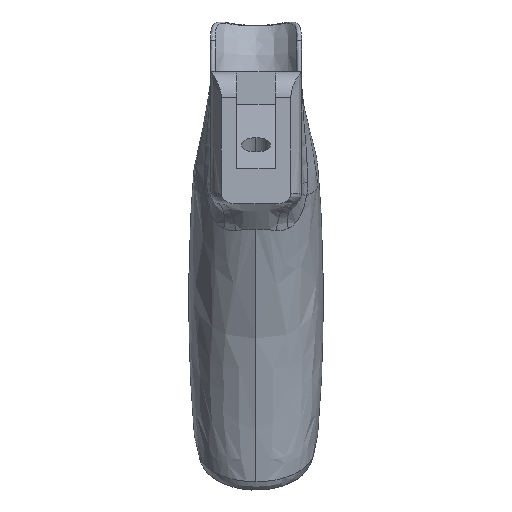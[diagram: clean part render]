
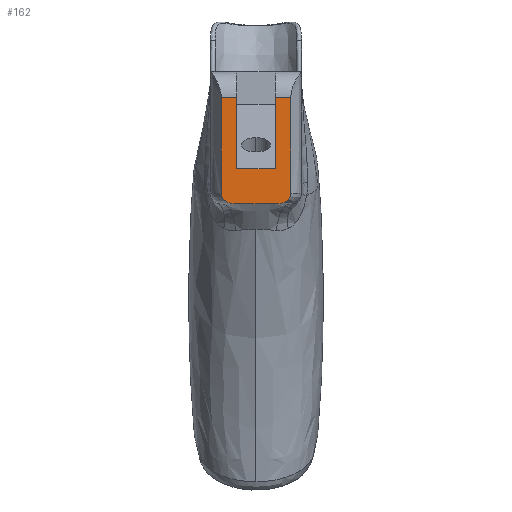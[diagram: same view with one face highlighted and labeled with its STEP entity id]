
A CAD part, top view. The second image highlights one B-rep face of the part: STEP entity #162.
In plain terms, the highlighted planar face has unit normal (0, 0, 1).
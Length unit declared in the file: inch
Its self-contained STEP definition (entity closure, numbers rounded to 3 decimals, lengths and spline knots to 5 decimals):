
#19 = VECTOR ( 'NONE', #7024, 39.37008 ) ;
#74 = CARTESIAN_POINT ( 'NONE',  ( -0.24455, -1.27484, 0. ) ) ;
#162 = ADVANCED_FACE ( 'NONE', ( #7116 ), #1725, .T. ) ;
#166 = VECTOR ( 'NONE', #4047, 39.37008 ) ;
#286 = CARTESIAN_POINT ( 'NONE',  ( 0.3375, -1.1789, 0. ) ) ;
#316 = VECTOR ( 'NONE', #1721, 39.37008 ) ;
#456 = DIRECTION ( 'NONE',  ( 0., 1., 0. ) ) ;
#489 = CARTESIAN_POINT ( 'NONE',  ( -0.188, -0.94, 0. ) ) ;
#516 = CARTESIAN_POINT ( 'NONE',  ( -0.188, -0.25, 0. ) ) ;
#560 = CARTESIAN_POINT ( 'NONE',  ( -0.26647, -1.26868, 0. ) ) ;
#705 = ORIENTED_EDGE ( 'NONE', *, *, #6036, .T. ) ;
#712 = CARTESIAN_POINT ( 'NONE',  ( -0.2069, -1.2789, 0. ) ) ;
#732 = CARTESIAN_POINT ( 'NONE',  ( 0.3208, -1.22844, 0. ) ) ;
#767 = ORIENTED_EDGE ( 'NONE', *, *, #5271, .F. ) ;
#1080 = DIRECTION ( 'NONE',  ( 1., 0., 0. ) ) ;
#1212 = LINE ( 'NONE', #3583, #316 ) ;
#1233 = CARTESIAN_POINT ( 'NONE',  ( -0.32073, -1.22843, 0. ) ) ;
#1303 = CARTESIAN_POINT ( 'NONE',  ( -0.30517, -1.2451, 0. ) ) ;
#1326 = CARTESIAN_POINT ( 'NONE',  ( 0.30534, -1.24507, 0. ) ) ;
#1360 = B_SPLINE_CURVE_WITH_KNOTS ( 'NONE', 3,
 ( #3565, #4887, #5471, #6614, #1813, #1233, #4848, #1303, #6647, #5400, #560, #74, #1739, #2376, #5361, #6543 ),
 .UNSPECIFIED., .F., .F.,
 ( 4, 2, 2, 2, 2, 2, 2, 4 ),
 ( 0., 0.00058, 0.00115, 0.00173, 0.0023, 0.00345, 0.00403, 0.0046 ),
 .UNSPECIFIED. ) ;
#1496 = CARTESIAN_POINT ( 'NONE',  ( -0.3375, -0.25, 0. ) ) ;
#1583 = ORIENTED_EDGE ( 'NONE', *, *, #2673, .F. ) ;
#1663 = VECTOR ( 'NONE', #2103, 39.37008 ) ;
#1671 = LINE ( 'NONE', #3535, #6327 ) ;
#1673 = VERTEX_POINT ( 'NONE', #2850 ) ;
#1721 = DIRECTION ( 'NONE',  ( 0., 1., 0. ) ) ;
#1725 = PLANE ( 'NONE',  #7564 ) ;
#1739 = CARTESIAN_POINT ( 'NONE',  ( -0.23707, -1.27637, 0. ) ) ;
#1784 = DIRECTION ( 'NONE',  ( 0., -1., 0. ) ) ;
#1805 = VECTOR ( 'NONE', #456, 39.37008 ) ;
#1813 = CARTESIAN_POINT ( 'NONE',  ( -0.32875, -1.21558, 0. ) ) ;
#1836 = DIRECTION ( 'NONE',  ( 0., -1., 0. ) ) ;
#1981 = CARTESIAN_POINT ( 'NONE',  ( 0.22262, -1.2789, 0. ) ) ;
#2103 = DIRECTION ( 'NONE',  ( 0., -1., 0. ) ) ;
#2192 = CARTESIAN_POINT ( 'NONE',  ( 0.20741, -1.2789, 0. ) ) ;
#2229 = ORIENTED_EDGE ( 'NONE', *, *, #2868, .F. ) ;
#2259 = LINE ( 'NONE', #7051, #6829 ) ;
#2285 = CARTESIAN_POINT ( 'NONE',  ( 0.3375, -0.25, 0. ) ) ;
#2314 = B_SPLINE_CURVE_WITH_KNOTS ( 'NONE', 3,
 ( #7379, #1981, #3261, #5649, #4285, #4906, #6710, #7295, #1326, #3735, #732, #3146, #5529, #2773, #5128, #286 ),
 .UNSPECIFIED., .F., .F.,
 ( 4, 2, 2, 2, 2, 2, 2, 4 ),
 ( 0., 0.00115, 0.00172, 0.00229, 0.00286, 0.00344, 0.00401, 0.00458 ),
 .UNSPECIFIED. ) ;
#2348 = CARTESIAN_POINT ( 'NONE',  ( 0.187, 0., 0. ) ) ;
#2376 = CARTESIAN_POINT ( 'NONE',  ( -0.22208, -1.27839, 0. ) ) ;
#2386 = DIRECTION ( 'NONE',  ( 1., 0., 0. ) ) ;
#2620 = ORIENTED_EDGE ( 'NONE', *, *, #2959, .T. ) ;
#2673 = EDGE_CURVE ( 'NONE', #3401, #3157, #5133, .T. ) ;
#2768 = VERTEX_POINT ( 'NONE', #2192 ) ;
#2773 = CARTESIAN_POINT ( 'NONE',  ( 0.33636, -1.19408, 0. ) ) ;
#2813 = VECTOR ( 'NONE', #1784, 39.37008 ) ;
#2850 = CARTESIAN_POINT ( 'NONE',  ( 0.187, -0.25, 0. ) ) ;
#2868 = EDGE_CURVE ( 'NONE', #1673, #3878, #5769, .T. ) ;
#2959 = EDGE_CURVE ( 'NONE', #4419, #3878, #5731, .T. ) ;
#3146 = CARTESIAN_POINT ( 'NONE',  ( 0.3288, -1.21555, 0. ) ) ;
#3157 = VERTEX_POINT ( 'NONE', #3578 ) ;
#3261 = CARTESIAN_POINT ( 'NONE',  ( 0.23752, -1.27691, 0. ) ) ;
#3335 = VERTEX_POINT ( 'NONE', #1496 ) ;
#3401 = VERTEX_POINT ( 'NONE', #516 ) ;
#3461 = CARTESIAN_POINT ( 'NONE',  ( -0.188, 0., 0. ) ) ;
#3535 = CARTESIAN_POINT ( 'NONE',  ( -0.4425, -0.25, 0. ) ) ;
#3565 = CARTESIAN_POINT ( 'NONE',  ( -0.3375, -1.1789, 0. ) ) ;
#3578 = CARTESIAN_POINT ( 'NONE',  ( -0.188, -0.94, 0. ) ) ;
#3583 = CARTESIAN_POINT ( 'NONE',  ( -0.3375, -1.2789, 0. ) ) ;
#3590 = CARTESIAN_POINT ( 'NONE',  ( -0.4425, -0.25, 0. ) ) ;
#3735 = CARTESIAN_POINT ( 'NONE',  ( 0.31598, -1.2344, 0. ) ) ;
#3784 = VERTEX_POINT ( 'NONE', #7038 ) ;
#3878 = VERTEX_POINT ( 'NONE', #2285 ) ;
#4047 = DIRECTION ( 'NONE',  ( 1., 0., 0. ) ) ;
#4093 = CARTESIAN_POINT ( 'NONE',  ( 0.3375, -1.2789, 0. ) ) ;
#4128 = LINE ( 'NONE', #489, #166 ) ;
#4152 = EDGE_LOOP ( 'NONE', ( #5767, #705, #2620, #2229, #6537, #767, #1583, #6741, #5642, #6626 ) ) ;
#4285 = CARTESIAN_POINT ( 'NONE',  ( 0.26655, -1.26818, 0. ) ) ;
#4419 = VERTEX_POINT ( 'NONE', #7027 ) ;
#4742 = EDGE_CURVE ( 'NONE', #6971, #2768, #2259, .T. ) ;
#4848 = CARTESIAN_POINT ( 'NONE',  ( -0.31587, -1.23443, 0. ) ) ;
#4887 = CARTESIAN_POINT ( 'NONE',  ( -0.3375, -1.18657, 0. ) ) ;
#4906 = CARTESIAN_POINT ( 'NONE',  ( 0.28026, -1.26198, 0. ) ) ;
#5019 = VERTEX_POINT ( 'NONE', #7173 ) ;
#5032 = EDGE_CURVE ( 'NONE', #1673, #3784, #6551, .T. ) ;
#5128 = CARTESIAN_POINT ( 'NONE',  ( 0.3375, -1.18656, 0. ) ) ;
#5133 = LINE ( 'NONE', #3461, #1663 ) ;
#5261 = EDGE_CURVE ( 'NONE', #3335, #3401, #1671, .T. ) ;
#5271 = EDGE_CURVE ( 'NONE', #3157, #3784, #4128, .T. ) ;
#5361 = CARTESIAN_POINT ( 'NONE',  ( -0.21452, -1.2789, 0. ) ) ;
#5400 = CARTESIAN_POINT ( 'NONE',  ( -0.28033, -1.26259, 0. ) ) ;
#5459 = EDGE_CURVE ( 'NONE', #5019, #6971, #1360, .T. ) ;
#5471 = CARTESIAN_POINT ( 'NONE',  ( -0.33636, -1.19404, 0. ) ) ;
#5529 = CARTESIAN_POINT ( 'NONE',  ( 0.33197, -1.20871, 0. ) ) ;
#5642 = ORIENTED_EDGE ( 'NONE', *, *, #5887, .F. ) ;
#5649 = CARTESIAN_POINT ( 'NONE',  ( 0.25938, -1.27077, 0. ) ) ;
#5731 = LINE ( 'NONE', #4093, #1805 ) ;
#5767 = ORIENTED_EDGE ( 'NONE', *, *, #4742, .T. ) ;
#5769 = LINE ( 'NONE', #5850, #19 ) ;
#5850 = CARTESIAN_POINT ( 'NONE',  ( -0.4425, -0.25, 0. ) ) ;
#5887 = EDGE_CURVE ( 'NONE', #5019, #3335, #1212, .T. ) ;
#6036 = EDGE_CURVE ( 'NONE', #2768, #4419, #2314, .T. ) ;
#6327 = VECTOR ( 'NONE', #2386, 39.37008 ) ;
#6537 = ORIENTED_EDGE ( 'NONE', *, *, #5032, .T. ) ;
#6543 = CARTESIAN_POINT ( 'NONE',  ( -0.2069, -1.2789, 0. ) ) ;
#6551 = LINE ( 'NONE', #2348, #2813 ) ;
#6614 = CARTESIAN_POINT ( 'NONE',  ( -0.33199, -1.20859, 0. ) ) ;
#6626 = ORIENTED_EDGE ( 'NONE', *, *, #5459, .T. ) ;
#6647 = CARTESIAN_POINT ( 'NONE',  ( -0.29931, -1.24986, 0. ) ) ;
#6710 = CARTESIAN_POINT ( 'NONE',  ( 0.28685, -1.25835, 0. ) ) ;
#6741 = ORIENTED_EDGE ( 'NONE', *, *, #5261, .F. ) ;
#6829 = VECTOR ( 'NONE', #1080, 39.37008 ) ;
#6971 = VERTEX_POINT ( 'NONE', #712 ) ;
#7024 = DIRECTION ( 'NONE',  ( 1., 0., 0. ) ) ;
#7027 = CARTESIAN_POINT ( 'NONE',  ( 0.3375, -1.1789, 0. ) ) ;
#7038 = CARTESIAN_POINT ( 'NONE',  ( 0.187, -0.94, 0. ) ) ;
#7051 = CARTESIAN_POINT ( 'NONE',  ( -0.4425, -1.2789, 0. ) ) ;
#7116 = FACE_OUTER_BOUND ( 'NONE', #4152, .T. ) ;
#7173 = CARTESIAN_POINT ( 'NONE',  ( -0.3375, -1.1789, 0. ) ) ;
#7263 = DIRECTION ( 'NONE',  ( 0., 0., 1. ) ) ;
#7295 = CARTESIAN_POINT ( 'NONE',  ( 0.29941, -1.24989, 0. ) ) ;
#7379 = CARTESIAN_POINT ( 'NONE',  ( 0.20741, -1.2789, 0. ) ) ;
#7564 = AXIS2_PLACEMENT_3D ( 'NONE', #3590, #7263, #1836 ) ;
